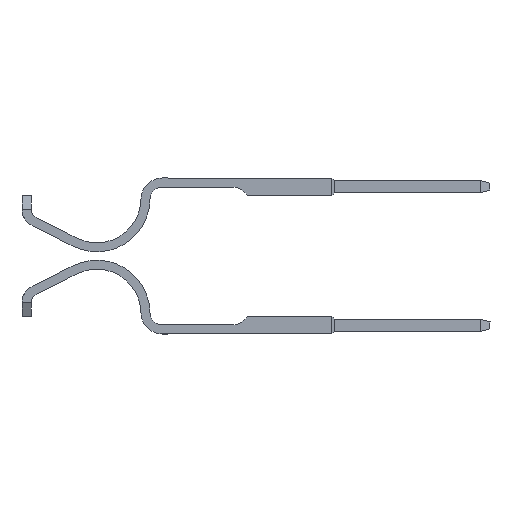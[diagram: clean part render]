
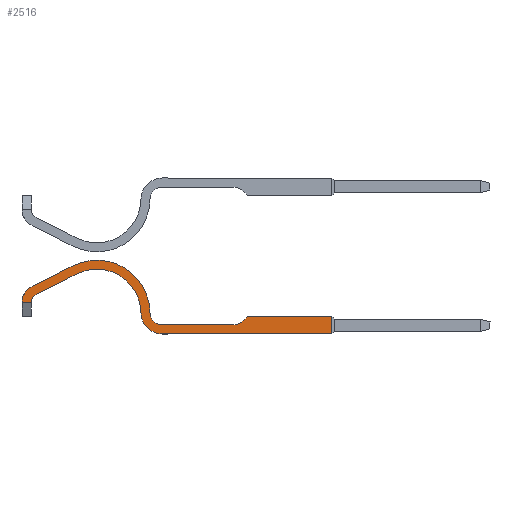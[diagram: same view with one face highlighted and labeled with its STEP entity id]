
A CAD part, left-side view. The second image highlights one B-rep face of the part: STEP entity #2516.
In plain terms, the highlighted face is planar.
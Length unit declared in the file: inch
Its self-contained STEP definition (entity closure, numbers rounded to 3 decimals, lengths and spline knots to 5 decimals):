
#166 = EDGE_CURVE ( 'NONE', #23092, #12011, #4078, .T. ) ;
#295 = ORIENTED_EDGE ( 'NONE', *, *, #15806, .F. ) ;
#707 = EDGE_CURVE ( 'NONE', #14165, #21372, #19767, .T. ) ;
#806 = VERTEX_POINT ( 'NONE', #6617 ) ;
#880 = DIRECTION ( 'NONE',  ( 0., 0., -1. ) ) ;
#882 = ORIENTED_EDGE ( 'NONE', *, *, #12534, .F. ) ;
#1201 = CARTESIAN_POINT ( 'NONE',  ( 0.58021, 0.0375, 0.025 ) ) ;
#1423 = PLANE ( 'NONE',  #3437 ) ;
#1426 = DIRECTION ( 'NONE',  ( 0., 0., -1. ) ) ;
#1544 = CARTESIAN_POINT ( 'NONE',  ( 0.43721, 0.04723, 0.025 ) ) ;
#1592 = VECTOR ( 'NONE', #14231, 39.37008 ) ;
#2210 = ORIENTED_EDGE ( 'NONE', *, *, #7911, .T. ) ;
#2217 = DIRECTION ( 'NONE',  ( 1., 0., 0. ) ) ;
#2228 = CARTESIAN_POINT ( 'NONE',  ( 0.15365, 0.06956, 0.025 ) ) ;
#2363 = ORIENTED_EDGE ( 'NONE', *, *, #9538, .T. ) ;
#2377 = EDGE_CURVE ( 'NONE', #8592, #21372, #9963, .T. ) ;
#2516 = ADVANCED_FACE ( 'NONE', ( #8904 ), #1423, .F. ) ;
#2859 = AXIS2_PLACEMENT_3D ( 'NONE', #22454, #11500, #7936 ) ;
#3437 = AXIS2_PLACEMENT_3D ( 'NONE', #12337, #16174, #15920 ) ;
#3716 = LINE ( 'NONE', #5463, #6230 ) ;
#3899 = CARTESIAN_POINT ( 'NONE',  ( 0.45258, 0.03186, 0.025 ) ) ;
#4078 = CIRCLE ( 'NONE', #4450, 0.0265 ) ;
#4450 = AXIS2_PLACEMENT_3D ( 'NONE', #10617, #19947, #21810 ) ;
#4709 = VECTOR ( 'NONE', #5958, 39.37008 ) ;
#4908 = CARTESIAN_POINT ( 'NONE',  ( 0.14621, 0.058, 0.025 ) ) ;
#5064 = EDGE_LOOP ( 'NONE', ( #9664, #2210, #23218, #2363, #16495, #20854, #17829, #22529, #15595, #23099, #21033, #9168, #295, #882, #9090 ) ) ;
#5111 = DIRECTION ( 'NONE',  ( 1., 0., 0. ) ) ;
#5329 = CARTESIAN_POINT ( 'NONE',  ( 0.58021, 0.0375, 0.025 ) ) ;
#5463 = CARTESIAN_POINT ( 'NONE',  ( 0.45821, 0.0375, 0.025 ) ) ;
#5958 = DIRECTION ( 'NONE',  ( -0.707, -0.707, 0. ) ) ;
#6230 = VECTOR ( 'NONE', #21882, 39.37008 ) ;
#6397 = DIRECTION ( 'NONE',  ( 1., 0., 0. ) ) ;
#6536 = DIRECTION ( 'NONE',  ( -1., 0., 0. ) ) ;
#6617 = CARTESIAN_POINT ( 'NONE',  ( 0.30469, 0.0435, 0.025 ) ) ;
#6655 = CARTESIAN_POINT ( 'NONE',  ( 0.15971, 0.0575, 0.025 ) ) ;
#6807 = CIRCLE ( 'NONE', #10993, 0.0185 ) ;
#7131 = CARTESIAN_POINT ( 'NONE',  ( 0.45821, 0.0375, 0.025 ) ) ;
#7873 = LINE ( 'NONE', #9316, #22127 ) ;
#7911 = EDGE_CURVE ( 'NONE', #23092, #13564, #21331, .T. ) ;
#7936 = DIRECTION ( 'NONE',  ( 1., 0., 0. ) ) ;
#8592 = VERTEX_POINT ( 'NONE', #12971 ) ;
#8764 = VERTEX_POINT ( 'NONE', #10344 ) ;
#8851 = CARTESIAN_POINT ( 'NONE',  ( 0.14781, 0.08118, 0.025 ) ) ;
#8904 = FACE_OUTER_BOUND ( 'NONE', #5064, .T. ) ;
#9090 = ORIENTED_EDGE ( 'NONE', *, *, #12389, .F. ) ;
#9168 = ORIENTED_EDGE ( 'NONE', *, *, #19301, .F. ) ;
#9177 = CARTESIAN_POINT ( 'NONE',  ( 0.45821, 0.0375, 0.025 ) ) ;
#9178 = VERTEX_POINT ( 'NONE', #10392 ) ;
#9305 = LINE ( 'NONE', #9177, #4709 ) ;
#9316 = CARTESIAN_POINT ( 'NONE',  ( 0.33619, 0.0255, 0.025 ) ) ;
#9447 = DIRECTION ( 'NONE',  ( -1., 0., 0. ) ) ;
#9538 = EDGE_CURVE ( 'NONE', #22259, #21815, #16866, .T. ) ;
#9664 = ORIENTED_EDGE ( 'NONE', *, *, #166, .F. ) ;
#9963 = LINE ( 'NONE', #22701, #22028 ) ;
#10051 = EDGE_CURVE ( 'NONE', #18140, #11228, #17070, .T. ) ;
#10344 = CARTESIAN_POINT ( 'NONE',  ( 0.20684, 0.11085, 0.025 ) ) ;
#10392 = CARTESIAN_POINT ( 'NONE',  ( 0.31769, 0.04371, 0.025 ) ) ;
#10600 = DIRECTION ( 'NONE',  ( 1., 0., 0. ) ) ;
#10617 = CARTESIAN_POINT ( 'NONE',  ( 0.15971, 0.0575, 0.025 ) ) ;
#10661 = DIRECTION ( 'NONE',  ( 0., -1., 0. ) ) ;
#10843 = EDGE_CURVE ( 'NONE', #21815, #806, #17997, .T. ) ;
#10993 = AXIS2_PLACEMENT_3D ( 'NONE', #16566, #14873, #14752 ) ;
#11223 = CARTESIAN_POINT ( 'NONE',  ( 0.2412, 0.0425, 0.025 ) ) ;
#11228 = VERTEX_POINT ( 'NONE', #11899 ) ;
#11236 = DIRECTION ( 'NONE',  ( 0.893, 0.449, 0. ) ) ;
#11500 = DIRECTION ( 'NONE',  ( 0., 0., 1. ) ) ;
#11585 = CARTESIAN_POINT ( 'NONE',  ( 0.2412, 0.0425, 0.025 ) ) ;
#11692 = VECTOR ( 'NONE', #11236, 39.37008 ) ;
#11899 = CARTESIAN_POINT ( 'NONE',  ( 0.43721, 0.0255, 0.025 ) ) ;
#12011 = VERTEX_POINT ( 'NONE', #13581 ) ;
#12158 = LINE ( 'NONE', #8851, #1592 ) ;
#12337 = CARTESIAN_POINT ( 'NONE',  ( 0.095, 0.025, 0.025 ) ) ;
#12389 = EDGE_CURVE ( 'NONE', #12011, #8764, #12158, .T. ) ;
#12534 = EDGE_CURVE ( 'NONE', #8764, #9178, #13755, .T. ) ;
#12971 = CARTESIAN_POINT ( 'NONE',  ( 0.33619, 0.0125, 0.025 ) ) ;
#13283 = CARTESIAN_POINT ( 'NONE',  ( 0.15365, 0.06956, 0.025 ) ) ;
#13368 = EDGE_CURVE ( 'NONE', #14165, #17067, #3716, .T. ) ;
#13417 = AXIS2_PLACEMENT_3D ( 'NONE', #11585, #15514, #20782 ) ;
#13556 = EDGE_CURVE ( 'NONE', #806, #8592, #13877, .T. ) ;
#13564 = VERTEX_POINT ( 'NONE', #17251 ) ;
#13581 = CARTESIAN_POINT ( 'NONE',  ( 0.14781, 0.08118, 0.025 ) ) ;
#13647 = CARTESIAN_POINT ( 'NONE',  ( 0.33619, 0.0255, 0.025 ) ) ;
#13729 = CARTESIAN_POINT ( 'NONE',  ( 0.13322, 0.058, 0.025 ) ) ;
#13755 = CIRCLE ( 'NONE', #20247, 0.0765 ) ;
#13877 = CIRCLE ( 'NONE', #2859, 0.0315 ) ;
#14165 = VERTEX_POINT ( 'NONE', #1201 ) ;
#14231 = DIRECTION ( 'NONE',  ( 0.893, 0.449, 0. ) ) ;
#14752 = DIRECTION ( 'NONE',  ( 1., 0., 0. ) ) ;
#14853 = CARTESIAN_POINT ( 'NONE',  ( 0.58021, 0.0125, 0.025 ) ) ;
#14873 = DIRECTION ( 'NONE',  ( 0., 0., 1. ) ) ;
#15479 = VECTOR ( 'NONE', #10661, 39.37008 ) ;
#15514 = DIRECTION ( 'NONE',  ( 0., 0., -1. ) ) ;
#15595 = ORIENTED_EDGE ( 'NONE', *, *, #13368, .T. ) ;
#15806 = EDGE_CURVE ( 'NONE', #9178, #16369, #6807, .T. ) ;
#15920 = DIRECTION ( 'NONE',  ( -1., 0., 0. ) ) ;
#16174 = DIRECTION ( 'NONE',  ( 0., 0., -1. ) ) ;
#16369 = VERTEX_POINT ( 'NONE', #13647 ) ;
#16495 = ORIENTED_EDGE ( 'NONE', *, *, #10843, .T. ) ;
#16511 = VECTOR ( 'NONE', #10600, 39.37008 ) ;
#16566 = CARTESIAN_POINT ( 'NONE',  ( 0.33619, 0.044, 0.025 ) ) ;
#16866 = LINE ( 'NONE', #13283, #11692 ) ;
#17067 = VERTEX_POINT ( 'NONE', #7131 ) ;
#17070 = CIRCLE ( 'NONE', #17845, 0.02173 ) ;
#17251 = CARTESIAN_POINT ( 'NONE',  ( 0.14622, 0.058, 0.025 ) ) ;
#17631 = AXIS2_PLACEMENT_3D ( 'NONE', #6655, #880, #6536 ) ;
#17829 = ORIENTED_EDGE ( 'NONE', *, *, #2377, .T. ) ;
#17845 = AXIS2_PLACEMENT_3D ( 'NONE', #1544, #1426, #5111 ) ;
#17997 = CIRCLE ( 'NONE', #13417, 0.0635 ) ;
#18029 = CIRCLE ( 'NONE', #17631, 0.0135 ) ;
#18140 = VERTEX_POINT ( 'NONE', #3899 ) ;
#18527 = DIRECTION ( 'NONE',  ( 0., 0., -1. ) ) ;
#19301 = EDGE_CURVE ( 'NONE', #16369, #11228, #7873, .T. ) ;
#19767 = LINE ( 'NONE', #5329, #15479 ) ;
#19947 = DIRECTION ( 'NONE',  ( 0., 0., -1. ) ) ;
#20247 = AXIS2_PLACEMENT_3D ( 'NONE', #11223, #18527, #9447 ) ;
#20650 = EDGE_CURVE ( 'NONE', #13564, #22259, #18029, .T. ) ;
#20782 = DIRECTION ( 'NONE',  ( -1., 0., 0. ) ) ;
#20854 = ORIENTED_EDGE ( 'NONE', *, *, #13556, .T. ) ;
#21033 = ORIENTED_EDGE ( 'NONE', *, *, #10051, .T. ) ;
#21331 = LINE ( 'NONE', #4908, #16511 ) ;
#21372 = VERTEX_POINT ( 'NONE', #14853 ) ;
#21810 = DIRECTION ( 'NONE',  ( -1., 0., 0. ) ) ;
#21815 = VERTEX_POINT ( 'NONE', #22420 ) ;
#21882 = DIRECTION ( 'NONE',  ( -1., 0., 0. ) ) ;
#22028 = VECTOR ( 'NONE', #6397, 39.37008 ) ;
#22127 = VECTOR ( 'NONE', #2217, 39.37008 ) ;
#22259 = VERTEX_POINT ( 'NONE', #2228 ) ;
#22420 = CARTESIAN_POINT ( 'NONE',  ( 0.21268, 0.09924, 0.025 ) ) ;
#22454 = CARTESIAN_POINT ( 'NONE',  ( 0.33619, 0.044, 0.025 ) ) ;
#22529 = ORIENTED_EDGE ( 'NONE', *, *, #707, .F. ) ;
#22701 = CARTESIAN_POINT ( 'NONE',  ( 0.33619, 0.0125, 0.025 ) ) ;
#23092 = VERTEX_POINT ( 'NONE', #13729 ) ;
#23099 = ORIENTED_EDGE ( 'NONE', *, *, #23361, .T. ) ;
#23218 = ORIENTED_EDGE ( 'NONE', *, *, #20650, .T. ) ;
#23361 = EDGE_CURVE ( 'NONE', #17067, #18140, #9305, .T. ) ;
